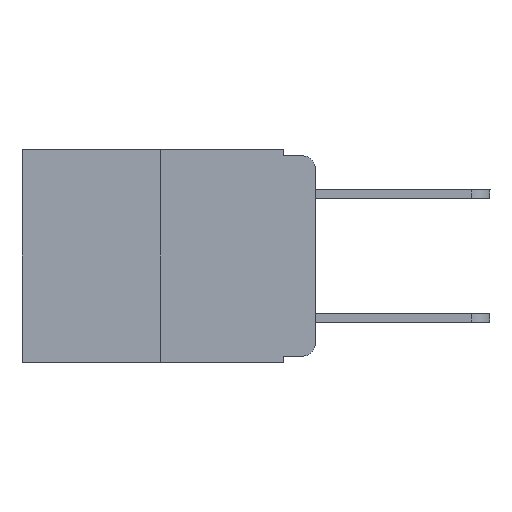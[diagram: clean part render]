
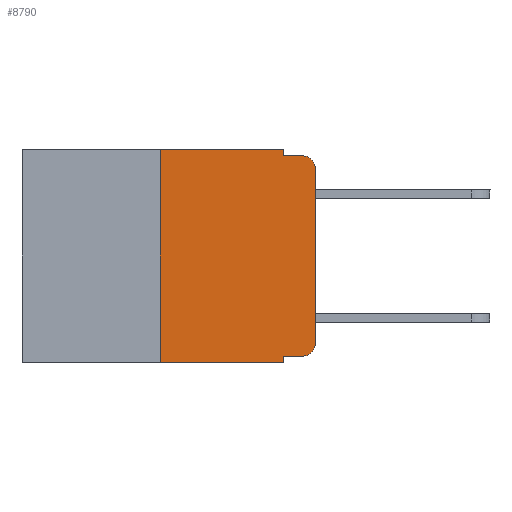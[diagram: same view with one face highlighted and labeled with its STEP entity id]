
A CAD part, left-side view. The second image highlights one B-rep face of the part: STEP entity #8790.
In plain terms, the highlighted planar face has unit normal (-1, 0, 0).
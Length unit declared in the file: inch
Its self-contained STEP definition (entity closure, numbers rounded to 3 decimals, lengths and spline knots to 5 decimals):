
#53 = CARTESIAN_POINT ( 'NONE',  ( 0., 0.051, -0.343 ) ) ;
#58 = CARTESIAN_POINT ( 'NONE',  ( 0., 0.051, 0. ) ) ;
#66 = CARTESIAN_POINT ( 'NONE',  ( 0., 0., -0.313 ) ) ;
#711 = DIRECTION ( 'NONE',  ( 0., 0., -1. ) ) ;
#916 = VERTEX_POINT ( 'NONE', #5988 ) ;
#1152 = EDGE_LOOP ( 'NONE', ( #6794, #7280, #9894, #1837, #7049, #6761, #13414, #4622, #3414, #4863 ) ) ;
#1626 = DIRECTION ( 'NONE',  ( 0., 0., 1. ) ) ;
#1692 = CARTESIAN_POINT ( 'NONE',  ( 0., 0., 0. ) ) ;
#1837 = ORIENTED_EDGE ( 'NONE', *, *, #4115, .F. ) ;
#2073 = DIRECTION ( 'NONE',  ( 1., 0., 0. ) ) ;
#2183 = VECTOR ( 'NONE', #7198, 39.37008 ) ;
#2241 = DIRECTION ( 'NONE',  ( 0., 0., -1. ) ) ;
#2323 = VECTOR ( 'NONE', #8369, 39.37008 ) ;
#2575 = VERTEX_POINT ( 'NONE', #13208 ) ;
#2749 = DIRECTION ( 'NONE',  ( 0., -1., 0. ) ) ;
#2793 = VERTEX_POINT ( 'NONE', #53 ) ;
#2804 = LINE ( 'NONE', #6161, #2183 ) ;
#2838 = CARTESIAN_POINT ( 'NONE',  ( 0., 0.051, 0. ) ) ;
#3161 = LINE ( 'NONE', #9721, #3823 ) ;
#3410 = VERTEX_POINT ( 'NONE', #8766 ) ;
#3414 = ORIENTED_EDGE ( 'NONE', *, *, #4165, .T. ) ;
#3517 = VECTOR ( 'NONE', #711, 39.37008 ) ;
#3528 = CARTESIAN_POINT ( 'NONE',  ( 0., 0.25, 0. ) ) ;
#3549 = EDGE_CURVE ( 'NONE', #916, #7474, #11169, .T. ) ;
#3823 = VECTOR ( 'NONE', #7435, 39.37008 ) ;
#4029 = CARTESIAN_POINT ( 'NONE',  ( 0., 0.051, -0.333 ) ) ;
#4076 = DIRECTION ( 'NONE',  ( 0., 0., -1. ) ) ;
#4115 = EDGE_CURVE ( 'NONE', #8038, #2575, #4171, .T. ) ;
#4165 = EDGE_CURVE ( 'NONE', #5685, #11050, #11148, .T. ) ;
#4171 = LINE ( 'NONE', #58, #2323 ) ;
#4379 = PLANE ( 'NONE',  #7861 ) ;
#4622 = ORIENTED_EDGE ( 'NONE', *, *, #12125, .F. ) ;
#4863 = ORIENTED_EDGE ( 'NONE', *, *, #11499, .T. ) ;
#5253 = VERTEX_POINT ( 'NONE', #9302 ) ;
#5472 = EDGE_CURVE ( 'NONE', #2575, #3410, #3161, .T. ) ;
#5618 = EDGE_CURVE ( 'NONE', #7474, #8038, #10874, .T. ) ;
#5649 = CIRCLE ( 'NONE', #8058, 0.02 ) ;
#5685 = VERTEX_POINT ( 'NONE', #4029 ) ;
#5988 = CARTESIAN_POINT ( 'NONE',  ( 0., 0.25, -0.343 ) ) ;
#6036 = CARTESIAN_POINT ( 'NONE',  ( 0., 0.051, 0. ) ) ;
#6161 = CARTESIAN_POINT ( 'NONE',  ( 0., 0.473, -0.343 ) ) ;
#6761 = ORIENTED_EDGE ( 'NONE', *, *, #3549, .F. ) ;
#6767 = LINE ( 'NONE', #1692, #8315 ) ;
#6768 = CARTESIAN_POINT ( 'NONE',  ( 0., 0.25, 0. ) ) ;
#6794 = ORIENTED_EDGE ( 'NONE', *, *, #11120, .T. ) ;
#7049 = ORIENTED_EDGE ( 'NONE', *, *, #5618, .F. ) ;
#7126 = VECTOR ( 'NONE', #11934, 39.37008 ) ;
#7198 = DIRECTION ( 'NONE',  ( 0., -1., 0. ) ) ;
#7231 = CIRCLE ( 'NONE', #12511, 0.02 ) ;
#7280 = ORIENTED_EDGE ( 'NONE', *, *, #7566, .T. ) ;
#7406 = CARTESIAN_POINT ( 'NONE',  ( 0., 0.02, -0.333 ) ) ;
#7435 = DIRECTION ( 'NONE',  ( 0., -1., 0. ) ) ;
#7474 = VERTEX_POINT ( 'NONE', #6768 ) ;
#7488 = CARTESIAN_POINT ( 'NONE',  ( 0., 0.051, -0.333 ) ) ;
#7527 = DIRECTION ( 'NONE',  ( -1., 0., 0. ) ) ;
#7566 = EDGE_CURVE ( 'NONE', #5253, #3410, #5649, .T. ) ;
#7861 = AXIS2_PLACEMENT_3D ( 'NONE', #11489, #2073, #9977 ) ;
#8038 = VERTEX_POINT ( 'NONE', #2838 ) ;
#8058 = AXIS2_PLACEMENT_3D ( 'NONE', #10431, #13452, #4076 ) ;
#8315 = VECTOR ( 'NONE', #1626, 39.37008 ) ;
#8369 = DIRECTION ( 'NONE',  ( 0., 0., -1. ) ) ;
#8766 = CARTESIAN_POINT ( 'NONE',  ( 0., 0.02, -0.01 ) ) ;
#8790 = ADVANCED_FACE ( 'NONE', ( #11695 ), #4379, .F. ) ;
#8901 = VECTOR ( 'NONE', #12918, 39.37008 ) ;
#9302 = CARTESIAN_POINT ( 'NONE',  ( 0., 0., -0.03 ) ) ;
#9351 = VECTOR ( 'NONE', #2749, 39.37008 ) ;
#9721 = CARTESIAN_POINT ( 'NONE',  ( 0., 0.051, -0.01 ) ) ;
#9792 = LINE ( 'NONE', #6036, #3517 ) ;
#9894 = ORIENTED_EDGE ( 'NONE', *, *, #5472, .F. ) ;
#9977 = DIRECTION ( 'NONE',  ( 0., 0., -1. ) ) ;
#10267 = EDGE_CURVE ( 'NONE', #916, #2793, #2804, .T. ) ;
#10431 = CARTESIAN_POINT ( 'NONE',  ( 0., 0.02, -0.03 ) ) ;
#10874 = LINE ( 'NONE', #12939, #9351 ) ;
#11050 = VERTEX_POINT ( 'NONE', #7406 ) ;
#11120 = EDGE_CURVE ( 'NONE', #12312, #5253, #6767, .T. ) ;
#11148 = LINE ( 'NONE', #7488, #8901 ) ;
#11169 = LINE ( 'NONE', #3528, #7126 ) ;
#11489 = CARTESIAN_POINT ( 'NONE',  ( 0., 0.473, 0. ) ) ;
#11499 = EDGE_CURVE ( 'NONE', #11050, #12312, #7231, .T. ) ;
#11695 = FACE_OUTER_BOUND ( 'NONE', #1152, .T. ) ;
#11934 = DIRECTION ( 'NONE',  ( 0., 0., 1. ) ) ;
#12125 = EDGE_CURVE ( 'NONE', #5685, #2793, #9792, .T. ) ;
#12312 = VERTEX_POINT ( 'NONE', #66 ) ;
#12511 = AXIS2_PLACEMENT_3D ( 'NONE', #12894, #7527, #2241 ) ;
#12894 = CARTESIAN_POINT ( 'NONE',  ( 0., 0.02, -0.313 ) ) ;
#12918 = DIRECTION ( 'NONE',  ( 0., -1., 0. ) ) ;
#12939 = CARTESIAN_POINT ( 'NONE',  ( 0., 0.473, 0. ) ) ;
#13208 = CARTESIAN_POINT ( 'NONE',  ( 0., 0.051, -0.01 ) ) ;
#13414 = ORIENTED_EDGE ( 'NONE', *, *, #10267, .T. ) ;
#13452 = DIRECTION ( 'NONE',  ( -1., 0., 0. ) ) ;
